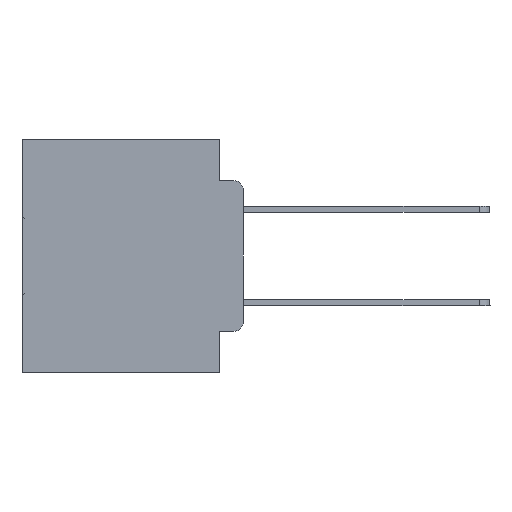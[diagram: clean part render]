
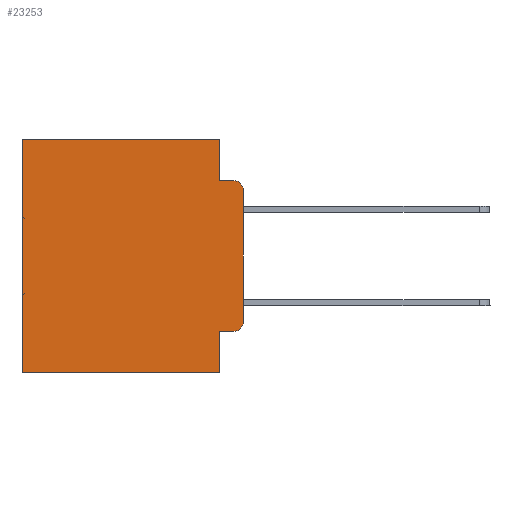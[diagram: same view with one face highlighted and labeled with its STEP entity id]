
A CAD part, left-side view. The second image highlights one B-rep face of the part: STEP entity #23253.
In plain terms, the highlighted planar face has unit normal (-1, 0, 0).
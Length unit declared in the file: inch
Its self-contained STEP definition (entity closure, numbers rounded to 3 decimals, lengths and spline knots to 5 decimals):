
#445 = VERTEX_POINT ( 'NONE', #11277 ) ;
#1559 = LINE ( 'NONE', #25827, #15483 ) ;
#1826 = VERTEX_POINT ( 'NONE', #30878 ) ;
#2849 = VECTOR ( 'NONE', #25225, 39.37008 ) ;
#3446 = VECTOR ( 'NONE', #15375, 39.37008 ) ;
#5265 = CARTESIAN_POINT ( 'NONE',  ( 0.298, 0.02, -0.0885 ) ) ;
#5540 = VERTEX_POINT ( 'NONE', #23367 ) ;
#6048 = CARTESIAN_POINT ( 'NONE',  ( 0.298, 0., -0.1085 ) ) ;
#6812 = EDGE_CURVE ( 'NONE', #24983, #33813, #13385, .T. ) ;
#7421 = VECTOR ( 'NONE', #27379, 39.37008 ) ;
#7472 = VECTOR ( 'NONE', #8491, 39.37008 ) ;
#8248 = EDGE_CURVE ( 'NONE', #5540, #22497, #9032, .T. ) ;
#8312 = EDGE_CURVE ( 'NONE', #24983, #22497, #28074, .T. ) ;
#8491 = DIRECTION ( 'NONE',  ( 0., 0., -1. ) ) ;
#8825 = ORIENTED_EDGE ( 'NONE', *, *, #8248, .F. ) ;
#9032 = LINE ( 'NONE', #11745, #2849 ) ;
#9149 = EDGE_CURVE ( 'NONE', #33978, #15244, #32111, .T. ) ;
#9645 = DIRECTION ( 'NONE',  ( 0., 0., -1. ) ) ;
#9743 = CARTESIAN_POINT ( 'NONE',  ( 0.298, 0.473, 0. ) ) ;
#11277 = CARTESIAN_POINT ( 'NONE',  ( 0.298, 0.02, -0.4115 ) ) ;
#11646 = CARTESIAN_POINT ( 'NONE',  ( 0.298, 0.02, -0.3915 ) ) ;
#11694 = CARTESIAN_POINT ( 'NONE',  ( 0.298, 0.051, 0. ) ) ;
#11745 = CARTESIAN_POINT ( 'NONE',  ( 0.298, 0.051, -0.0885 ) ) ;
#11881 = ORIENTED_EDGE ( 'NONE', *, *, #6812, .F. ) ;
#11992 = DIRECTION ( 'NONE',  ( 0., -1., 0. ) ) ;
#12026 = LINE ( 'NONE', #25684, #34551 ) ;
#12076 = LINE ( 'NONE', #19631, #7472 ) ;
#12879 = ORIENTED_EDGE ( 'NONE', *, *, #18836, .F. ) ;
#13044 = CARTESIAN_POINT ( 'NONE',  ( 0.298, 0., 0. ) ) ;
#13385 = LINE ( 'NONE', #16057, #7421 ) ;
#13662 = CARTESIAN_POINT ( 'NONE',  ( 0.298, 0.051, -0.5 ) ) ;
#13932 = CIRCLE ( 'NONE', #30595, 0.02 ) ;
#14176 = LINE ( 'NONE', #22257, #23404 ) ;
#15047 = DIRECTION ( 'NONE',  ( 1., 0., 0. ) ) ;
#15244 = VERTEX_POINT ( 'NONE', #9743 ) ;
#15375 = DIRECTION ( 'NONE',  ( 0., 1., 0. ) ) ;
#15483 = VECTOR ( 'NONE', #11992, 39.37008 ) ;
#15692 = ORIENTED_EDGE ( 'NONE', *, *, #24498, .F. ) ;
#16057 = CARTESIAN_POINT ( 'NONE',  ( 0.298, 0., 0. ) ) ;
#17306 = EDGE_CURVE ( 'NONE', #15244, #19668, #14176, .T. ) ;
#17750 = DIRECTION ( 'NONE',  ( -1., 0., 0. ) ) ;
#17869 = ORIENTED_EDGE ( 'NONE', *, *, #8312, .T. ) ;
#18836 = EDGE_CURVE ( 'NONE', #33978, #5540, #33477, .T. ) ;
#19621 = ORIENTED_EDGE ( 'NONE', *, *, #17306, .T. ) ;
#19631 = CARTESIAN_POINT ( 'NONE',  ( 0.298, 0.051, 0. ) ) ;
#19668 = VERTEX_POINT ( 'NONE', #28254 ) ;
#19740 = ORIENTED_EDGE ( 'NONE', *, *, #33207, .T. ) ;
#20106 = EDGE_LOOP ( 'NONE', ( #11881, #17869, #8825, #12879, #27890, #19621, #15692, #30931, #28058, #19740 ) ) ;
#20615 = PLANE ( 'NONE',  #32842 ) ;
#20667 = EDGE_CURVE ( 'NONE', #1826, #445, #1559, .T. ) ;
#20715 = DIRECTION ( 'NONE',  ( 0., 0., -1. ) ) ;
#22257 = CARTESIAN_POINT ( 'NONE',  ( 0.298, 0.473, 0. ) ) ;
#22497 = VERTEX_POINT ( 'NONE', #5265 ) ;
#22976 = DIRECTION ( 'NONE',  ( 0., 1., 0. ) ) ;
#23050 = CARTESIAN_POINT ( 'NONE',  ( 0.298, 0.02, -0.1085 ) ) ;
#23253 = ADVANCED_FACE ( 'NONE', ( #23663 ), #20615, .F. ) ;
#23367 = CARTESIAN_POINT ( 'NONE',  ( 0.298, 0.051, -0.0885 ) ) ;
#23404 = VECTOR ( 'NONE', #25134, 39.37008 ) ;
#23663 = FACE_OUTER_BOUND ( 'NONE', #20106, .T. ) ;
#24498 = EDGE_CURVE ( 'NONE', #28323, #19668, #12026, .T. ) ;
#24983 = VERTEX_POINT ( 'NONE', #6048 ) ;
#25134 = DIRECTION ( 'NONE',  ( 0., 0., -1. ) ) ;
#25225 = DIRECTION ( 'NONE',  ( 0., -1., 0. ) ) ;
#25684 = CARTESIAN_POINT ( 'NONE',  ( 0.298, 0., -0.5 ) ) ;
#25827 = CARTESIAN_POINT ( 'NONE',  ( 0.298, 0.051, -0.4115 ) ) ;
#26018 = CARTESIAN_POINT ( 'NONE',  ( 0.298, 0., 0. ) ) ;
#27379 = DIRECTION ( 'NONE',  ( 0., 0., -1. ) ) ;
#27890 = ORIENTED_EDGE ( 'NONE', *, *, #9149, .T. ) ;
#27999 = VECTOR ( 'NONE', #30424, 39.37008 ) ;
#28058 = ORIENTED_EDGE ( 'NONE', *, *, #20667, .T. ) ;
#28074 = CIRCLE ( 'NONE', #28658, 0.02 ) ;
#28254 = CARTESIAN_POINT ( 'NONE',  ( 0.298, 0.473, -0.5 ) ) ;
#28323 = VERTEX_POINT ( 'NONE', #13662 ) ;
#28658 = AXIS2_PLACEMENT_3D ( 'NONE', #23050, #31700, #20715 ) ;
#28723 = DIRECTION ( 'NONE',  ( 0., 0., -1. ) ) ;
#30064 = CARTESIAN_POINT ( 'NONE',  ( 0.298, 0., -0.3915 ) ) ;
#30424 = DIRECTION ( 'NONE',  ( 0., 0., -1. ) ) ;
#30595 = AXIS2_PLACEMENT_3D ( 'NONE', #11646, #17750, #28723 ) ;
#30878 = CARTESIAN_POINT ( 'NONE',  ( 0.298, 0.051, -0.4115 ) ) ;
#30931 = ORIENTED_EDGE ( 'NONE', *, *, #31115, .F. ) ;
#31115 = EDGE_CURVE ( 'NONE', #1826, #28323, #12076, .T. ) ;
#31700 = DIRECTION ( 'NONE',  ( -1., 0., 0. ) ) ;
#32111 = LINE ( 'NONE', #13044, #3446 ) ;
#32842 = AXIS2_PLACEMENT_3D ( 'NONE', #26018, #15047, #9645 ) ;
#33207 = EDGE_CURVE ( 'NONE', #445, #33813, #13932, .T. ) ;
#33477 = LINE ( 'NONE', #33647, #27999 ) ;
#33647 = CARTESIAN_POINT ( 'NONE',  ( 0.298, 0.051, 0. ) ) ;
#33813 = VERTEX_POINT ( 'NONE', #30064 ) ;
#33978 = VERTEX_POINT ( 'NONE', #11694 ) ;
#34551 = VECTOR ( 'NONE', #22976, 39.37008 ) ;
